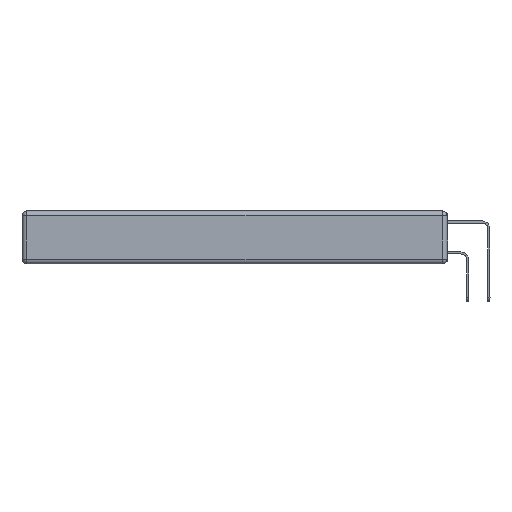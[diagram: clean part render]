
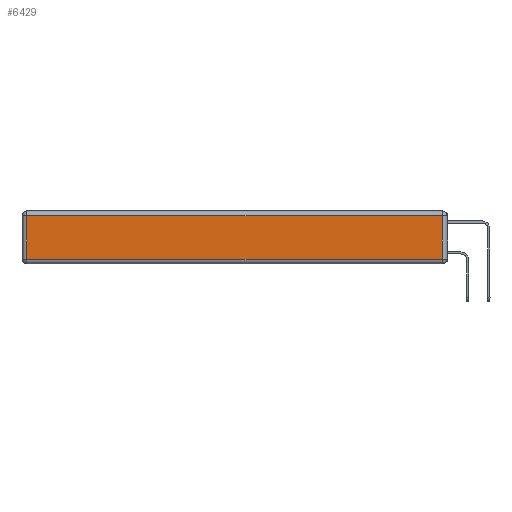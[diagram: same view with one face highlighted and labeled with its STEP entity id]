
A CAD part, left-side view. The second image highlights one B-rep face of the part: STEP entity #6429.
In plain terms, the highlighted planar face has unit normal (-1, 0, 0).
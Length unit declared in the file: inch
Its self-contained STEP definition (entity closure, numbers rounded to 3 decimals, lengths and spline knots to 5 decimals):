
#629 = CARTESIAN_POINT ( 'NONE',  ( 0., 0., -0.313 ) ) ;
#919 = EDGE_LOOP ( 'NONE', ( #16689, #10850, #1281, #4135 ) ) ;
#1281 = ORIENTED_EDGE ( 'NONE', *, *, #2948, .T. ) ;
#1460 = DIRECTION ( 'NONE',  ( 0., 0., -1. ) ) ;
#2212 = DIRECTION ( 'NONE',  ( 0., -1., 0. ) ) ;
#2645 = CARTESIAN_POINT ( 'NONE',  ( 0., 0., -0.343 ) ) ;
#2948 = EDGE_CURVE ( 'NONE', #16500, #13670, #12190, .T. ) ;
#3179 = EDGE_CURVE ( 'NONE', #13625, #16774, #17461, .T. ) ;
#3834 = DIRECTION ( 'NONE',  ( -1., 0., 0. ) ) ;
#4135 = ORIENTED_EDGE ( 'NONE', *, *, #9629, .T. ) ;
#4180 = VECTOR ( 'NONE', #6449, 39.37008 ) ;
#4372 = CARTESIAN_POINT ( 'NONE',  ( 0., 0.03, -0.03 ) ) ;
#5418 = FACE_OUTER_BOUND ( 'NONE', #919, .T. ) ;
#6159 = CARTESIAN_POINT ( 'NONE',  ( 0., 2.75, -0.03 ) ) ;
#6429 = ADVANCED_FACE ( 'NONE', ( #5418 ), #11278, .T. ) ;
#6449 = DIRECTION ( 'NONE',  ( 0., 1., 0. ) ) ;
#7853 = DIRECTION ( 'NONE',  ( 0., 0., 1. ) ) ;
#9105 = LINE ( 'NONE', #10477, #18566 ) ;
#9629 = EDGE_CURVE ( 'NONE', #13670, #13625, #9105, .T. ) ;
#10192 = AXIS2_PLACEMENT_3D ( 'NONE', #2645, #3834, #17427 ) ;
#10477 = CARTESIAN_POINT ( 'NONE',  ( 0., 2.72, -0.343 ) ) ;
#10719 = CARTESIAN_POINT ( 'NONE',  ( 0., 0.03, -0.313 ) ) ;
#10850 = ORIENTED_EDGE ( 'NONE', *, *, #18871, .T. ) ;
#10854 = CARTESIAN_POINT ( 'NONE',  ( 0., 2.72, -0.313 ) ) ;
#11278 = PLANE ( 'NONE',  #10192 ) ;
#11999 = VECTOR ( 'NONE', #2212, 39.37008 ) ;
#12190 = LINE ( 'NONE', #6159, #4180 ) ;
#13079 = VECTOR ( 'NONE', #7853, 39.37008 ) ;
#13625 = VERTEX_POINT ( 'NONE', #10854 ) ;
#13670 = VERTEX_POINT ( 'NONE', #13681 ) ;
#13681 = CARTESIAN_POINT ( 'NONE',  ( 0., 2.72, -0.03 ) ) ;
#15269 = CARTESIAN_POINT ( 'NONE',  ( 0., 0.03, -0.343 ) ) ;
#16500 = VERTEX_POINT ( 'NONE', #4372 ) ;
#16689 = ORIENTED_EDGE ( 'NONE', *, *, #3179, .T. ) ;
#16774 = VERTEX_POINT ( 'NONE', #10719 ) ;
#17427 = DIRECTION ( 'NONE',  ( 0., 0., 1. ) ) ;
#17461 = LINE ( 'NONE', #629, #11999 ) ;
#18405 = LINE ( 'NONE', #15269, #13079 ) ;
#18566 = VECTOR ( 'NONE', #1460, 39.37008 ) ;
#18871 = EDGE_CURVE ( 'NONE', #16774, #16500, #18405, .T. ) ;
